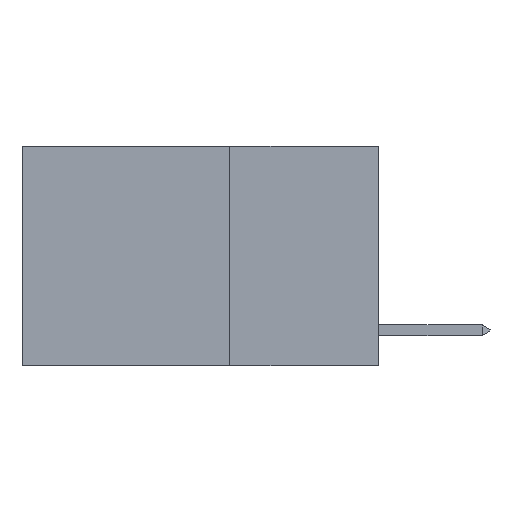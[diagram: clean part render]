
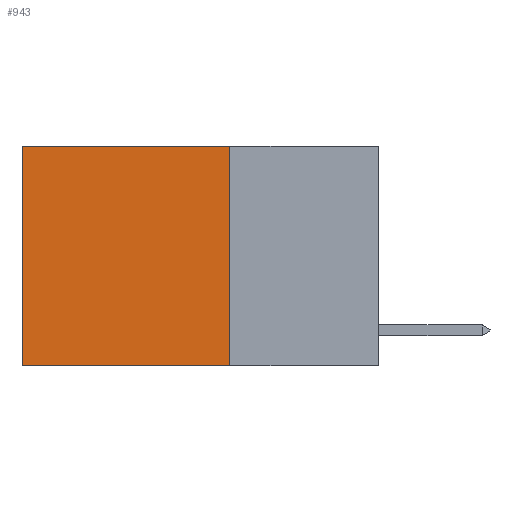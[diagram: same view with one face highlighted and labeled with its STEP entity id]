
A CAD part, left-side view. The second image highlights one B-rep face of the part: STEP entity #943.
In plain terms, the highlighted planar face has unit normal (-1, 0, 0).
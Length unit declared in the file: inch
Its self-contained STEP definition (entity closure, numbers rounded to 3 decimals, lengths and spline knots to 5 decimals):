
#442 = CARTESIAN_POINT ( 'NONE',  ( 0.2625, 0.25, 0. ) ) ;
#483 = LINE ( 'NONE', #1188, #9812 ) ;
#578 = DIRECTION ( 'NONE',  ( 1., 0., 0. ) ) ;
#715 = EDGE_CURVE ( 'NONE', #5900, #5503, #9054, .T. ) ;
#943 = ADVANCED_FACE ( 'NONE', ( #8173 ), #1336, .F. ) ;
#1010 = ORIENTED_EDGE ( 'NONE', *, *, #7189, .T. ) ;
#1188 = CARTESIAN_POINT ( 'NONE',  ( 0.2625, 0.25, -0.37 ) ) ;
#1284 = DIRECTION ( 'NONE',  ( 0., 1., 0. ) ) ;
#1301 = ORIENTED_EDGE ( 'NONE', *, *, #3755, .F. ) ;
#1336 = PLANE ( 'NONE',  #7884 ) ;
#1366 = DIRECTION ( 'NONE',  ( 0., 0., -1. ) ) ;
#2080 = LINE ( 'NONE', #8114, #7507 ) ;
#2331 = DIRECTION ( 'NONE',  ( 0., 1., 0. ) ) ;
#2432 = LINE ( 'NONE', #9228, #7225 ) ;
#2665 = VERTEX_POINT ( 'NONE', #7716 ) ;
#2779 = EDGE_LOOP ( 'NONE', ( #4363, #1301, #8333, #1010 ) ) ;
#3755 = EDGE_CURVE ( 'NONE', #2665, #5503, #483, .T. ) ;
#4341 = EDGE_CURVE ( 'NONE', #4469, #2665, #2080, .T. ) ;
#4363 = ORIENTED_EDGE ( 'NONE', *, *, #715, .T. ) ;
#4469 = VERTEX_POINT ( 'NONE', #4483 ) ;
#4483 = CARTESIAN_POINT ( 'NONE',  ( 0.2625, 0.25, 0. ) ) ;
#5503 = VERTEX_POINT ( 'NONE', #7764 ) ;
#5900 = VERTEX_POINT ( 'NONE', #6962 ) ;
#6687 = DIRECTION ( 'NONE',  ( 0., 0., -1. ) ) ;
#6962 = CARTESIAN_POINT ( 'NONE',  ( 0.2625, 0.6, 0. ) ) ;
#7104 = VECTOR ( 'NONE', #9289, 39.37008 ) ;
#7189 = EDGE_CURVE ( 'NONE', #4469, #5900, #2432, .T. ) ;
#7225 = VECTOR ( 'NONE', #2331, 39.37008 ) ;
#7507 = VECTOR ( 'NONE', #1366, 39.37008 ) ;
#7716 = CARTESIAN_POINT ( 'NONE',  ( 0.2625, 0.25, -0.37 ) ) ;
#7764 = CARTESIAN_POINT ( 'NONE',  ( 0.2625, 0.6, -0.37 ) ) ;
#7781 = CARTESIAN_POINT ( 'NONE',  ( 0.2625, 0.6, 0. ) ) ;
#7884 = AXIS2_PLACEMENT_3D ( 'NONE', #442, #578, #6687 ) ;
#8114 = CARTESIAN_POINT ( 'NONE',  ( 0.2625, 0.25, 0. ) ) ;
#8173 = FACE_OUTER_BOUND ( 'NONE', #2779, .T. ) ;
#8333 = ORIENTED_EDGE ( 'NONE', *, *, #4341, .F. ) ;
#9054 = LINE ( 'NONE', #7781, #7104 ) ;
#9228 = CARTESIAN_POINT ( 'NONE',  ( 0.2625, 0.25, 0. ) ) ;
#9289 = DIRECTION ( 'NONE',  ( 0., 0., -1. ) ) ;
#9812 = VECTOR ( 'NONE', #1284, 39.37008 ) ;
